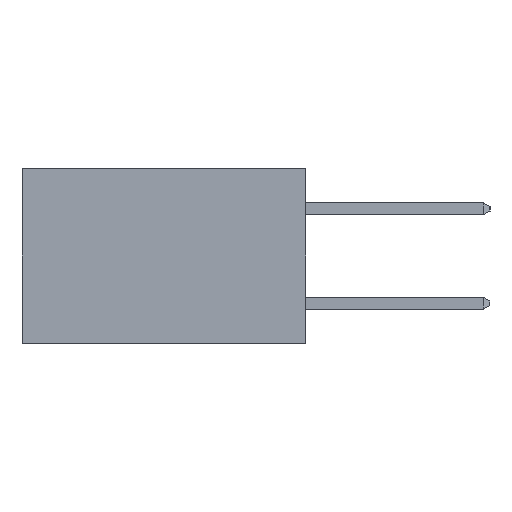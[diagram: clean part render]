
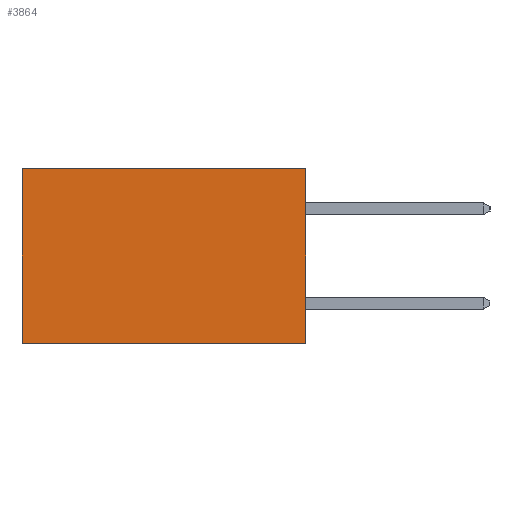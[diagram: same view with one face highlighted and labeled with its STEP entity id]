
A CAD part, left-side view. The second image highlights one B-rep face of the part: STEP entity #3864.
In plain terms, the highlighted planar face has unit normal (-1, 0, 0).
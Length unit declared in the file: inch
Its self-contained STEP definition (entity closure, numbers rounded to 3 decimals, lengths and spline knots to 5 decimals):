
#871 = ORIENTED_EDGE ( 'NONE', *, *, #15789, .T. ) ;
#974 = CARTESIAN_POINT ( 'NONE',  ( 0.298, 0.6, -0.37 ) ) ;
#1160 = EDGE_CURVE ( 'NONE', #15347, #12033, #18449, .T. ) ;
#2524 = EDGE_LOOP ( 'NONE', ( #17292, #17555, #17793, #871 ) ) ;
#3038 = VERTEX_POINT ( 'NONE', #10232 ) ;
#3864 = ADVANCED_FACE ( 'NONE', ( #7398 ), #14208, .F. ) ;
#4805 = CARTESIAN_POINT ( 'NONE',  ( 0.298, 0., -0.37 ) ) ;
#5717 = CARTESIAN_POINT ( 'NONE',  ( 0.298, 0., 0. ) ) ;
#7398 = FACE_OUTER_BOUND ( 'NONE', #2524, .T. ) ;
#8151 = LINE ( 'NONE', #5717, #11608 ) ;
#8995 = EDGE_CURVE ( 'NONE', #3038, #12033, #10104, .T. ) ;
#9271 = CARTESIAN_POINT ( 'NONE',  ( 0.298, 0., 0. ) ) ;
#10104 = LINE ( 'NONE', #4805, #14110 ) ;
#10232 = CARTESIAN_POINT ( 'NONE',  ( 0.298, 0., -0.37 ) ) ;
#10776 = VECTOR ( 'NONE', #13177, 39.37008 ) ;
#11608 = VECTOR ( 'NONE', #21078, 39.37008 ) ;
#11740 = DIRECTION ( 'NONE',  ( 1., 0., 0. ) ) ;
#12033 = VERTEX_POINT ( 'NONE', #974 ) ;
#13177 = DIRECTION ( 'NONE',  ( 0., 0., -1. ) ) ;
#13307 = DIRECTION ( 'NONE',  ( 0., 1., 0. ) ) ;
#13870 = VECTOR ( 'NONE', #18880, 39.37008 ) ;
#14110 = VECTOR ( 'NONE', #13307, 39.37008 ) ;
#14208 = PLANE ( 'NONE',  #15821 ) ;
#15143 = VERTEX_POINT ( 'NONE', #9271 ) ;
#15347 = VERTEX_POINT ( 'NONE', #18371 ) ;
#15789 = EDGE_CURVE ( 'NONE', #15143, #15347, #8151, .T. ) ;
#15821 = AXIS2_PLACEMENT_3D ( 'NONE', #17652, #11740, #20275 ) ;
#17292 = ORIENTED_EDGE ( 'NONE', *, *, #1160, .T. ) ;
#17555 = ORIENTED_EDGE ( 'NONE', *, *, #8995, .F. ) ;
#17652 = CARTESIAN_POINT ( 'NONE',  ( 0.298, 0., 0. ) ) ;
#17793 = ORIENTED_EDGE ( 'NONE', *, *, #21548, .F. ) ;
#18371 = CARTESIAN_POINT ( 'NONE',  ( 0.298, 0.6, 0. ) ) ;
#18449 = LINE ( 'NONE', #20225, #13870 ) ;
#18880 = DIRECTION ( 'NONE',  ( 0., 0., -1. ) ) ;
#19325 = LINE ( 'NONE', #21652, #10776 ) ;
#20225 = CARTESIAN_POINT ( 'NONE',  ( 0.298, 0.6, 0. ) ) ;
#20275 = DIRECTION ( 'NONE',  ( 0., 0., -1. ) ) ;
#21078 = DIRECTION ( 'NONE',  ( 0., 1., 0. ) ) ;
#21548 = EDGE_CURVE ( 'NONE', #15143, #3038, #19325, .T. ) ;
#21652 = CARTESIAN_POINT ( 'NONE',  ( 0.298, 0., 0. ) ) ;
